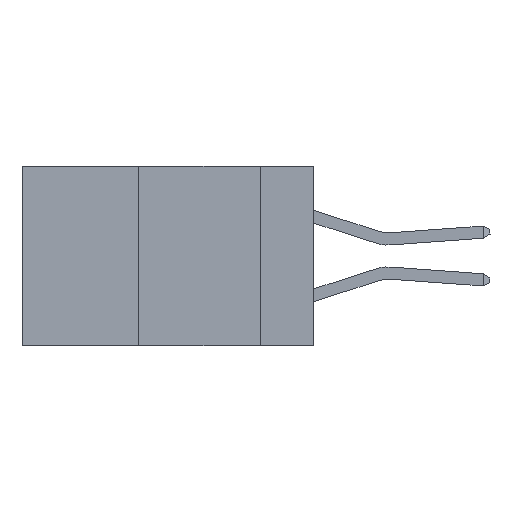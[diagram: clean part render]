
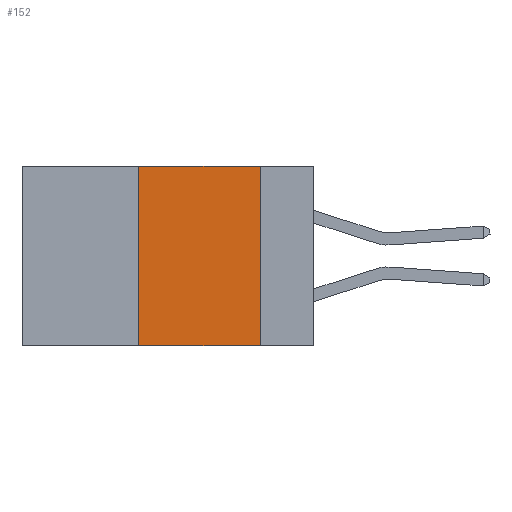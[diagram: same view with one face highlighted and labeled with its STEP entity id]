
A CAD part, left-side view. The second image highlights one B-rep face of the part: STEP entity #152.
In plain terms, the highlighted planar face has unit normal (-1, 0, 0).
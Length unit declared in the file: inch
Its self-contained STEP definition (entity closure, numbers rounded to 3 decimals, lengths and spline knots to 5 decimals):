
#124 = DIRECTION ( 'NONE',  ( 0., -1., 0. ) ) ;
#152 = ADVANCED_FACE ( 'NONE', ( #411 ), #8479, .F. ) ;
#381 = ORIENTED_EDGE ( 'NONE', *, *, #8467, .F. ) ;
#411 = FACE_OUTER_BOUND ( 'NONE', #3381, .T. ) ;
#671 = ORIENTED_EDGE ( 'NONE', *, *, #11999, .F. ) ;
#2482 = DIRECTION ( 'NONE',  ( 0., 0., -1. ) ) ;
#3381 = EDGE_LOOP ( 'NONE', ( #381, #11247, #671, #12223 ) ) ;
#3421 = CARTESIAN_POINT ( 'NONE',  ( 0., 0.11, -0.37 ) ) ;
#3753 = LINE ( 'NONE', #11505, #6478 ) ;
#4576 = AXIS2_PLACEMENT_3D ( 'NONE', #5626, #13729, #12032 ) ;
#5626 = CARTESIAN_POINT ( 'NONE',  ( 0., 0.6, 0. ) ) ;
#5832 = DIRECTION ( 'NONE',  ( 0., 0., 1. ) ) ;
#6478 = VECTOR ( 'NONE', #2482, 39.37008 ) ;
#6803 = CARTESIAN_POINT ( 'NONE',  ( 0., 0.11, 0. ) ) ;
#7063 = CARTESIAN_POINT ( 'NONE',  ( 0., 0.6, 0. ) ) ;
#8467 = EDGE_CURVE ( 'NONE', #14847, #11369, #3753, .T. ) ;
#8479 = PLANE ( 'NONE',  #4576 ) ;
#8480 = CARTESIAN_POINT ( 'NONE',  ( 0., 0.6, -0.37 ) ) ;
#8747 = LINE ( 'NONE', #7063, #11450 ) ;
#10196 = EDGE_CURVE ( 'NONE', #10639, #14847, #8747, .T. ) ;
#10255 = VECTOR ( 'NONE', #124, 39.37008 ) ;
#10639 = VERTEX_POINT ( 'NONE', #11425 ) ;
#10858 = CARTESIAN_POINT ( 'NONE',  ( 0., 0.36, -0.37 ) ) ;
#10981 = VERTEX_POINT ( 'NONE', #10858 ) ;
#11247 = ORIENTED_EDGE ( 'NONE', *, *, #10196, .F. ) ;
#11338 = VECTOR ( 'NONE', #5832, 39.37008 ) ;
#11369 = VERTEX_POINT ( 'NONE', #3421 ) ;
#11425 = CARTESIAN_POINT ( 'NONE',  ( 0., 0.36, 0. ) ) ;
#11450 = VECTOR ( 'NONE', #12737, 39.37008 ) ;
#11505 = CARTESIAN_POINT ( 'NONE',  ( 0., 0.11, 0. ) ) ;
#11646 = EDGE_CURVE ( 'NONE', #10981, #11369, #13578, .T. ) ;
#11999 = EDGE_CURVE ( 'NONE', #10981, #10639, #14237, .T. ) ;
#12032 = DIRECTION ( 'NONE',  ( 0., 0., -1. ) ) ;
#12223 = ORIENTED_EDGE ( 'NONE', *, *, #11646, .T. ) ;
#12737 = DIRECTION ( 'NONE',  ( 0., -1., 0. ) ) ;
#13578 = LINE ( 'NONE', #8480, #10255 ) ;
#13718 = CARTESIAN_POINT ( 'NONE',  ( 0., 0.36, 0. ) ) ;
#13729 = DIRECTION ( 'NONE',  ( 1., 0., 0. ) ) ;
#14237 = LINE ( 'NONE', #13718, #11338 ) ;
#14847 = VERTEX_POINT ( 'NONE', #6803 ) ;
